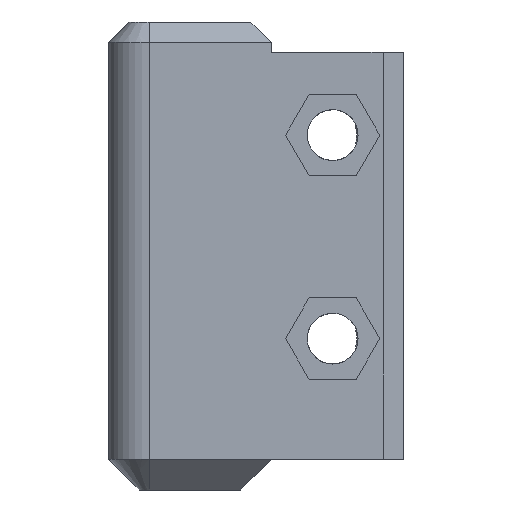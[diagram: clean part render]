
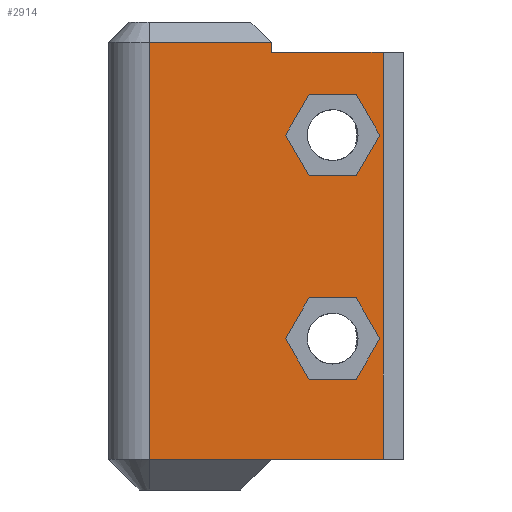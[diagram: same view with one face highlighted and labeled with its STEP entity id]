
A CAD part, front view. The second image highlights one B-rep face of the part: STEP entity #2914.
In plain terms, the highlighted planar face has unit normal (0, -1, 0).
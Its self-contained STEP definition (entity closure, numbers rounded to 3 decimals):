
#120=FACE_BOUND('',#1058,.T.);
#121=FACE_BOUND('',#1059,.T.);
#140=PLANE('',#3098);
#258=LINE('',#4207,#568);
#270=LINE('',#4239,#580);
#274=LINE('',#4248,#584);
#275=LINE('',#4250,#585);
#276=LINE('',#4252,#586);
#277=LINE('',#4254,#587);
#278=LINE('',#4256,#588);
#279=LINE('',#4258,#589);
#280=LINE('',#4259,#590);
#281=LINE('',#4260,#591);
#282=LINE('',#4263,#592);
#283=LINE('',#4265,#593);
#284=LINE('',#4267,#594);
#285=LINE('',#4269,#595);
#286=LINE('',#4271,#596);
#287=LINE('',#4272,#597);
#288=LINE('',#4275,#598);
#289=LINE('',#4277,#599);
#290=LINE('',#4279,#600);
#291=LINE('',#4281,#601);
#292=LINE('',#4283,#602);
#293=LINE('',#4284,#603);
#568=VECTOR('',#3370,10.);
#580=VECTOR('',#3400,10.);
#584=VECTOR('',#3408,10.);
#585=VECTOR('',#3409,10.);
#586=VECTOR('',#3410,1.);
#587=VECTOR('',#3411,10.);
#588=VECTOR('',#3412,10.);
#589=VECTOR('',#3413,10.);
#590=VECTOR('',#3414,10.);
#591=VECTOR('',#3415,4.);
#592=VECTOR('',#3416,10.);
#593=VECTOR('',#3417,10.);
#594=VECTOR('',#3418,10.);
#595=VECTOR('',#3419,10.);
#596=VECTOR('',#3420,10.);
#597=VECTOR('',#3421,10.);
#598=VECTOR('',#3422,10.);
#599=VECTOR('',#3423,10.);
#600=VECTOR('',#3424,10.);
#601=VECTOR('',#3425,10.);
#602=VECTOR('',#3426,10.);
#603=VECTOR('',#3427,10.);
#897=FACE_OUTER_BOUND('',#1057,.T.);
#1057=EDGE_LOOP('',(#2051,#2052,#2053,#2054,#2055,#2056,#2057,#2058,#2059,
#2060));
#1058=EDGE_LOOP('',(#2061,#2062,#2063,#2064,#2065,#2066));
#1059=EDGE_LOOP('',(#2067,#2068,#2069,#2070,#2071,#2072));
#1276=VERTEX_POINT('',#4200);
#1278=VERTEX_POINT('',#4205);
#1286=VERTEX_POINT('',#4229);
#1288=VERTEX_POINT('',#4235);
#1292=VERTEX_POINT('',#4247);
#1293=VERTEX_POINT('',#4249);
#1294=VERTEX_POINT('',#4251);
#1295=VERTEX_POINT('',#4253);
#1296=VERTEX_POINT('',#4255);
#1297=VERTEX_POINT('',#4257);
#1298=VERTEX_POINT('',#4261);
#1299=VERTEX_POINT('',#4262);
#1300=VERTEX_POINT('',#4264);
#1301=VERTEX_POINT('',#4266);
#1302=VERTEX_POINT('',#4268);
#1303=VERTEX_POINT('',#4270);
#1304=VERTEX_POINT('',#4273);
#1305=VERTEX_POINT('',#4274);
#1306=VERTEX_POINT('',#4276);
#1307=VERTEX_POINT('',#4278);
#1308=VERTEX_POINT('',#4280);
#1309=VERTEX_POINT('',#4282);
#1569=EDGE_CURVE('',#1278,#1276,#258,.T.);
#1585=EDGE_CURVE('',#1286,#1288,#270,.T.);
#1589=EDGE_CURVE('',#1278,#1292,#274,.T.);
#1590=EDGE_CURVE('',#1292,#1293,#275,.T.);
#1591=EDGE_CURVE('',#1293,#1294,#276,.T.);
#1592=EDGE_CURVE('',#1295,#1294,#277,.T.);
#1593=EDGE_CURVE('',#1296,#1295,#278,.T.);
#1594=EDGE_CURVE('',#1297,#1296,#279,.T.);
#1595=EDGE_CURVE('',#1288,#1297,#280,.T.);
#1596=EDGE_CURVE('',#1286,#1276,#281,.T.);
#1597=EDGE_CURVE('',#1298,#1299,#282,.T.);
#1598=EDGE_CURVE('',#1299,#1300,#283,.T.);
#1599=EDGE_CURVE('',#1300,#1301,#284,.T.);
#1600=EDGE_CURVE('',#1301,#1302,#285,.T.);
#1601=EDGE_CURVE('',#1302,#1303,#286,.T.);
#1602=EDGE_CURVE('',#1303,#1298,#287,.T.);
#1603=EDGE_CURVE('',#1304,#1305,#288,.T.);
#1604=EDGE_CURVE('',#1305,#1306,#289,.T.);
#1605=EDGE_CURVE('',#1306,#1307,#290,.T.);
#1606=EDGE_CURVE('',#1307,#1308,#291,.T.);
#1607=EDGE_CURVE('',#1308,#1309,#292,.T.);
#1608=EDGE_CURVE('',#1309,#1304,#293,.T.);
#2051=ORIENTED_EDGE('',*,*,#1569,.F.);
#2052=ORIENTED_EDGE('',*,*,#1589,.T.);
#2053=ORIENTED_EDGE('',*,*,#1590,.T.);
#2054=ORIENTED_EDGE('',*,*,#1591,.T.);
#2055=ORIENTED_EDGE('',*,*,#1592,.F.);
#2056=ORIENTED_EDGE('',*,*,#1593,.F.);
#2057=ORIENTED_EDGE('',*,*,#1594,.F.);
#2058=ORIENTED_EDGE('',*,*,#1595,.F.);
#2059=ORIENTED_EDGE('',*,*,#1585,.F.);
#2060=ORIENTED_EDGE('',*,*,#1596,.T.);
#2061=ORIENTED_EDGE('',*,*,#1597,.T.);
#2062=ORIENTED_EDGE('',*,*,#1598,.T.);
#2063=ORIENTED_EDGE('',*,*,#1599,.T.);
#2064=ORIENTED_EDGE('',*,*,#1600,.T.);
#2065=ORIENTED_EDGE('',*,*,#1601,.T.);
#2066=ORIENTED_EDGE('',*,*,#1602,.T.);
#2067=ORIENTED_EDGE('',*,*,#1603,.T.);
#2068=ORIENTED_EDGE('',*,*,#1604,.T.);
#2069=ORIENTED_EDGE('',*,*,#1605,.T.);
#2070=ORIENTED_EDGE('',*,*,#1606,.T.);
#2071=ORIENTED_EDGE('',*,*,#1607,.T.);
#2072=ORIENTED_EDGE('',*,*,#1608,.T.);
#2914=ADVANCED_FACE('',(#897,#120,#121),#140,.T.);
#3098=AXIS2_PLACEMENT_3D('',#4246,#3406,#3407);
#3370=DIRECTION('',(-1.,0.,0.));
#3400=DIRECTION('',(1.,0.,0.));
#3406=DIRECTION('center_axis',(0.,-1.,0.));
#3407=DIRECTION('ref_axis',(0.,0.,
-1.));
#3408=DIRECTION('',(0.,0.,1.));
#3409=DIRECTION('',(1.,0.,0.));
#3410=DIRECTION('',(1.,0.,0.));
#3411=DIRECTION('',(0.,0.,-1.));
#3412=DIRECTION('',(1.,0.,0.));
#3413=DIRECTION('',(1.,0.,0.));
#3414=DIRECTION('',(0.,0.,-1.));
#3415=DIRECTION('',(0.,0.,-1.));
#3416=DIRECTION('',(-0.5,0.,0.866));
#3417=DIRECTION('',(0.5,0.,0.866));
#3418=DIRECTION('',(1.,0.,0.));
#3419=DIRECTION('',(0.5,0.,-0.866));
#3420=DIRECTION('',(-0.5,0.,-0.866));
#3421=DIRECTION('',(-1.,0.,0.));
#3422=DIRECTION('',(-0.5,0.,0.866));
#3423=DIRECTION('',(0.5,0.,0.866));
#3424=DIRECTION('',(1.,0.,0.));
#3425=DIRECTION('',(0.5,0.,-0.866));
#3426=DIRECTION('',(-0.5,0.,-0.866));
#3427=DIRECTION('',(-1.,0.,0.));
#4200=CARTESIAN_POINT('',(2719.321,231.051,71.412));
#4205=CARTESIAN_POINT('',(2731.321,231.051,71.412));
#4207=CARTESIAN_POINT('',(2715.321,231.051,71.412));
#4229=CARTESIAN_POINT('',(2719.321,231.051,112.412));
#4235=CARTESIAN_POINT('',(2731.321,231.051,112.412));
#4239=CARTESIAN_POINT('',(2715.321,231.051,112.412));
#4246=CARTESIAN_POINT('Origin',(2715.321,231.051,114.412));
#4247=CARTESIAN_POINT('',(2731.321,231.051,71.439));
#4248=CARTESIAN_POINT('',(2731.321,231.051,102.912));
#4249=CARTESIAN_POINT('',(2736.65,231.051,71.439));
#4250=CARTESIAN_POINT('',(2724.565,231.051,71.44));
#4251=CARTESIAN_POINT('',(2742.31,231.051,71.439));
#4252=CARTESIAN_POINT('',(2744.31,231.051,71.439));
#4253=CARTESIAN_POINT('',(2742.31,231.051,111.439));
#4254=CARTESIAN_POINT('',(2742.31,231.051,102.687));
#4255=CARTESIAN_POINT('',(2736.651,231.051,111.439));
#4256=CARTESIAN_POINT('',(2735.481,231.051,111.439));
#4257=CARTESIAN_POINT('',(2731.321,231.051,111.439));
#4258=CARTESIAN_POINT('',(2725.316,231.051,111.44));
#4259=CARTESIAN_POINT('',(2731.321,231.051,102.912));
#4260=CARTESIAN_POINT('',(2719.321,231.051,102.912));
#4261=CARTESIAN_POINT('',(2735.034,231.051,99.283));
#4262=CARTESIAN_POINT('',(2732.719,231.051,103.293));
#4263=CARTESIAN_POINT('',(2728.137,231.051,111.229));
#4264=CARTESIAN_POINT('',(2735.034,231.051,107.303));
#4265=CARTESIAN_POINT('',(2734.109,231.051,105.701));
#4266=CARTESIAN_POINT('',(2739.664,231.051,107.303));
#4267=CARTESIAN_POINT('',(2727.492,231.051,107.303));
#4268=CARTESIAN_POINT('',(2741.979,231.051,103.293));
#4269=CARTESIAN_POINT('',(2736.24,231.051,113.234));
#4270=CARTESIAN_POINT('',(2739.664,231.051,99.283));
#4271=CARTESIAN_POINT('',(2739.897,231.051,99.686));
#4272=CARTESIAN_POINT('',(2725.177,231.051,99.283));
#4273=CARTESIAN_POINT('',(2735.033,231.051,79.283));
#4274=CARTESIAN_POINT('',(2732.718,231.051,83.293));
#4275=CARTESIAN_POINT('',(2723.806,231.051,98.729));
#4276=CARTESIAN_POINT('',(2735.033,231.051,87.303));
#4277=CARTESIAN_POINT('',(2738.439,231.051,93.201));
#4278=CARTESIAN_POINT('',(2739.664,231.051,87.303));
#4279=CARTESIAN_POINT('',(2727.492,231.051,87.303));
#4280=CARTESIAN_POINT('',(2741.979,231.051,83.293));
#4281=CARTESIAN_POINT('',(2731.909,231.051,100.734));
#4282=CARTESIAN_POINT('',(2739.664,231.051,79.283));
#4283=CARTESIAN_POINT('',(2744.226,231.051,87.186));
#4284=CARTESIAN_POINT('',(2725.177,231.051,79.283));
